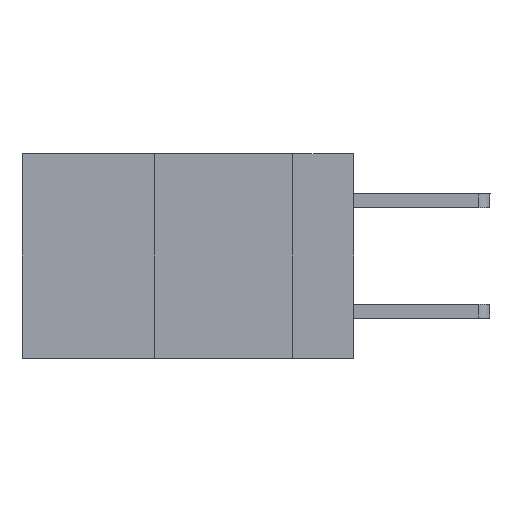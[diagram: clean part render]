
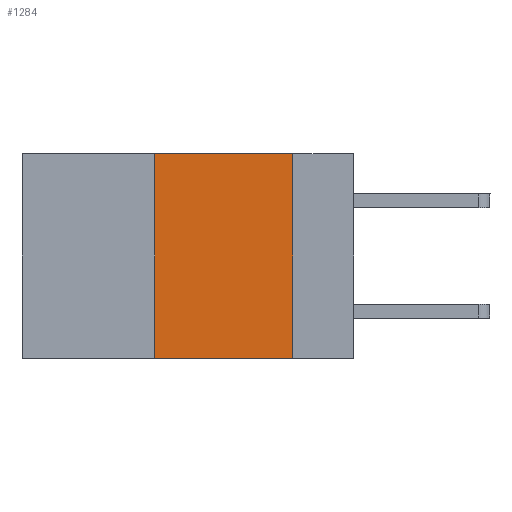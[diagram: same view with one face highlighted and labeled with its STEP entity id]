
A CAD part, left-side view. The second image highlights one B-rep face of the part: STEP entity #1284.
In plain terms, the highlighted planar face has unit normal (-1, 0, 0).
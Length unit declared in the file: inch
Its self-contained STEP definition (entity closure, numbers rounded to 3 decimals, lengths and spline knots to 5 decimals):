
#157 = CARTESIAN_POINT ( 'NONE',  ( 0., 0.6, -0.37 ) ) ;
#419 = CARTESIAN_POINT ( 'NONE',  ( 0., 0.6, 0. ) ) ;
#779 = VERTEX_POINT ( 'NONE', #2158 ) ;
#900 = AXIS2_PLACEMENT_3D ( 'NONE', #5718, #5005, #4934 ) ;
#1000 = PLANE ( 'NONE',  #900 ) ;
#1188 = CARTESIAN_POINT ( 'NONE',  ( 0., 0.36, 0. ) ) ;
#1284 = ADVANCED_FACE ( 'NONE', ( #8924 ), #1000, .F. ) ;
#1572 = LINE ( 'NONE', #157, #7522 ) ;
#2031 = EDGE_CURVE ( 'NONE', #5335, #6474, #2192, .T. ) ;
#2109 = ORIENTED_EDGE ( 'NONE', *, *, #9575, .F. ) ;
#2158 = CARTESIAN_POINT ( 'NONE',  ( 0., 0.11, -0.37 ) ) ;
#2192 = LINE ( 'NONE', #10079, #5048 ) ;
#2341 = EDGE_CURVE ( 'NONE', #5335, #779, #1572, .T. ) ;
#2540 = EDGE_CURVE ( 'NONE', #6474, #8492, #7396, .T. ) ;
#2575 = DIRECTION ( 'NONE',  ( 0., -1., 0. ) ) ;
#3061 = ORIENTED_EDGE ( 'NONE', *, *, #2031, .F. ) ;
#4934 = DIRECTION ( 'NONE',  ( 0., 0., -1. ) ) ;
#5005 = DIRECTION ( 'NONE',  ( 1., 0., 0. ) ) ;
#5048 = VECTOR ( 'NONE', #9383, 39.37008 ) ;
#5133 = EDGE_LOOP ( 'NONE', ( #2109, #7175, #3061, #8602 ) ) ;
#5144 = CARTESIAN_POINT ( 'NONE',  ( 0., 0.36, -0.37 ) ) ;
#5335 = VERTEX_POINT ( 'NONE', #5144 ) ;
#5381 = DIRECTION ( 'NONE',  ( 0., 0., -1. ) ) ;
#5486 = LINE ( 'NONE', #6178, #9353 ) ;
#5718 = CARTESIAN_POINT ( 'NONE',  ( 0., 0.6, 0. ) ) ;
#6178 = CARTESIAN_POINT ( 'NONE',  ( 0., 0.11, 0. ) ) ;
#6288 = CARTESIAN_POINT ( 'NONE',  ( 0., 0.11, 0. ) ) ;
#6474 = VERTEX_POINT ( 'NONE', #1188 ) ;
#7175 = ORIENTED_EDGE ( 'NONE', *, *, #2540, .F. ) ;
#7396 = LINE ( 'NONE', #419, #9287 ) ;
#7522 = VECTOR ( 'NONE', #2575, 39.37008 ) ;
#8492 = VERTEX_POINT ( 'NONE', #6288 ) ;
#8602 = ORIENTED_EDGE ( 'NONE', *, *, #2341, .T. ) ;
#8924 = FACE_OUTER_BOUND ( 'NONE', #5133, .T. ) ;
#9158 = DIRECTION ( 'NONE',  ( 0., -1., 0. ) ) ;
#9287 = VECTOR ( 'NONE', #9158, 39.37008 ) ;
#9353 = VECTOR ( 'NONE', #5381, 39.37008 ) ;
#9383 = DIRECTION ( 'NONE',  ( 0., 0., 1. ) ) ;
#9575 = EDGE_CURVE ( 'NONE', #8492, #779, #5486, .T. ) ;
#10079 = CARTESIAN_POINT ( 'NONE',  ( 0., 0.36, 0. ) ) ;
